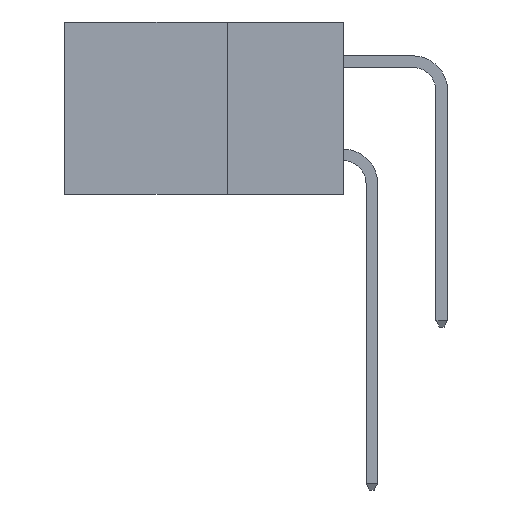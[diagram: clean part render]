
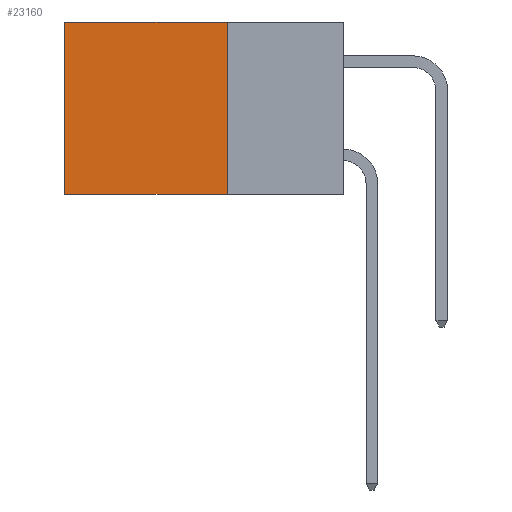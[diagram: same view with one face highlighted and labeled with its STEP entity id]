
A CAD part, left-side view. The second image highlights one B-rep face of the part: STEP entity #23160.
In plain terms, the highlighted planar face has unit normal (-1, 0, 0).
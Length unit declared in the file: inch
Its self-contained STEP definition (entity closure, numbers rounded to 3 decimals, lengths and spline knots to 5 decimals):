
#8 = VERTEX_POINT ( 'NONE', #14224 ) ;
#1713 = CARTESIAN_POINT ( 'NONE',  ( 0.2615, 0.6, 0. ) ) ;
#2917 = VECTOR ( 'NONE', #3844, 39.37008 ) ;
#3844 = DIRECTION ( 'NONE',  ( 0., 0., -1. ) ) ;
#4354 = VECTOR ( 'NONE', #8145, 39.37008 ) ;
#4658 = LINE ( 'NONE', #26694, #27320 ) ;
#4781 = VECTOR ( 'NONE', #26722, 39.37008 ) ;
#5929 = ORIENTED_EDGE ( 'NONE', *, *, #22598, .F. ) ;
#6592 = DIRECTION ( 'NONE',  ( 1., 0., 0. ) ) ;
#6881 = AXIS2_PLACEMENT_3D ( 'NONE', #19800, #6592, #21961 ) ;
#8145 = DIRECTION ( 'NONE',  ( 0., 1., 0. ) ) ;
#9289 = EDGE_CURVE ( 'NONE', #22052, #16630, #4658, .T. ) ;
#9539 = LINE ( 'NONE', #27941, #2917 ) ;
#11471 = CARTESIAN_POINT ( 'NONE',  ( 0.2615, 0.25, -0.37 ) ) ;
#11535 = DIRECTION ( 'NONE',  ( 0., 0., -1. ) ) ;
#13118 = FACE_OUTER_BOUND ( 'NONE', #20462, .T. ) ;
#14224 = CARTESIAN_POINT ( 'NONE',  ( 0.2615, 0.6, -0.37 ) ) ;
#15306 = CARTESIAN_POINT ( 'NONE',  ( 0.2615, 0.25, -0.37 ) ) ;
#16630 = VERTEX_POINT ( 'NONE', #15306 ) ;
#18134 = CARTESIAN_POINT ( 'NONE',  ( 0.2615, 0.25, 0. ) ) ;
#18396 = ORIENTED_EDGE ( 'NONE', *, *, #25110, .T. ) ;
#19800 = CARTESIAN_POINT ( 'NONE',  ( 0.2615, 0.25, -0.37 ) ) ;
#19820 = VERTEX_POINT ( 'NONE', #1713 ) ;
#20462 = EDGE_LOOP ( 'NONE', ( #18396, #5929, #21977, #25954 ) ) ;
#21677 = LINE ( 'NONE', #11471, #4781 ) ;
#21961 = DIRECTION ( 'NONE',  ( 0., 0., -1. ) ) ;
#21977 = ORIENTED_EDGE ( 'NONE', *, *, #9289, .F. ) ;
#22052 = VERTEX_POINT ( 'NONE', #18134 ) ;
#22598 = EDGE_CURVE ( 'NONE', #16630, #8, #21677, .T. ) ;
#23160 = ADVANCED_FACE ( 'NONE', ( #13118 ), #28393, .F. ) ;
#23703 = EDGE_CURVE ( 'NONE', #22052, #19820, #27022, .T. ) ;
#25110 = EDGE_CURVE ( 'NONE', #19820, #8, #9539, .T. ) ;
#25637 = CARTESIAN_POINT ( 'NONE',  ( 0.2615, 0.25, 0. ) ) ;
#25954 = ORIENTED_EDGE ( 'NONE', *, *, #23703, .T. ) ;
#26694 = CARTESIAN_POINT ( 'NONE',  ( 0.2615, 0.25, -0.37 ) ) ;
#26722 = DIRECTION ( 'NONE',  ( 0., 1., 0. ) ) ;
#27022 = LINE ( 'NONE', #25637, #4354 ) ;
#27320 = VECTOR ( 'NONE', #11535, 39.37008 ) ;
#27941 = CARTESIAN_POINT ( 'NONE',  ( 0.2615, 0.6, -0.37 ) ) ;
#28393 = PLANE ( 'NONE',  #6881 ) ;
